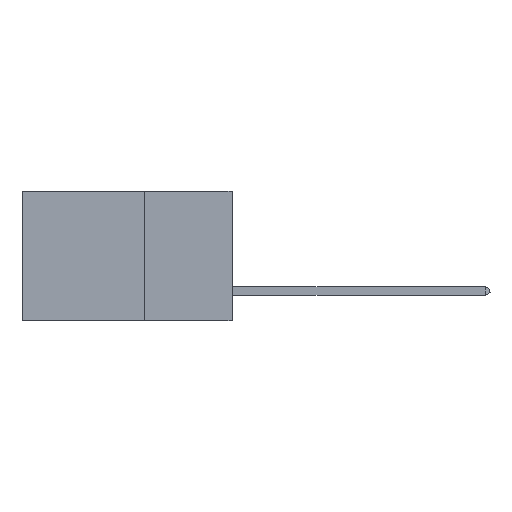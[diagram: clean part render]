
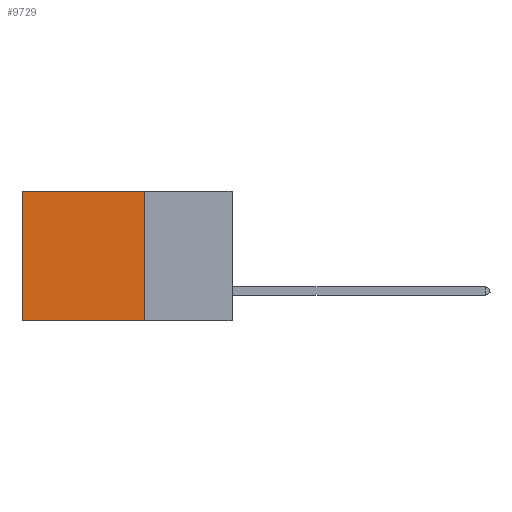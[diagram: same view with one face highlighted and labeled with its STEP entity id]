
A CAD part, left-side view. The second image highlights one B-rep face of the part: STEP entity #9729.
In plain terms, the highlighted planar face has unit normal (-1, 0, 0).
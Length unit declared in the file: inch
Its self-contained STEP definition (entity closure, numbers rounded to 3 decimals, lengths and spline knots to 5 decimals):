
#268 = VERTEX_POINT ( 'NONE', #613 ) ;
#613 = CARTESIAN_POINT ( 'NONE',  ( 0.2875, 0.6, 0. ) ) ;
#1703 = VERTEX_POINT ( 'NONE', #13849 ) ;
#1802 = CARTESIAN_POINT ( 'NONE',  ( 0.2875, 0.6, 0. ) ) ;
#2017 = CARTESIAN_POINT ( 'NONE',  ( 0.2875, 0.25, 0. ) ) ;
#2115 = AXIS2_PLACEMENT_3D ( 'NONE', #5458, #5613, #15082 ) ;
#3708 = VECTOR ( 'NONE', #10103, 39.37008 ) ;
#4011 = ORIENTED_EDGE ( 'NONE', *, *, #12187, .F. ) ;
#4267 = DIRECTION ( 'NONE',  ( 0., 1., 0. ) ) ;
#4859 = VECTOR ( 'NONE', #15124, 39.37008 ) ;
#5458 = CARTESIAN_POINT ( 'NONE',  ( 0.2875, 0.25, 0. ) ) ;
#5613 = DIRECTION ( 'NONE',  ( 1., 0., 0. ) ) ;
#6941 = VERTEX_POINT ( 'NONE', #2017 ) ;
#7247 = LINE ( 'NONE', #11249, #3708 ) ;
#8371 = VECTOR ( 'NONE', #4267, 39.37008 ) ;
#8663 = LINE ( 'NONE', #12694, #11103 ) ;
#8962 = EDGE_CURVE ( 'NONE', #6941, #11988, #8663, .T. ) ;
#9342 = ORIENTED_EDGE ( 'NONE', *, *, #12696, .T. ) ;
#9729 = ADVANCED_FACE ( 'NONE', ( #14822 ), #15032, .F. ) ;
#10103 = DIRECTION ( 'NONE',  ( 0., 1., 0. ) ) ;
#11071 = EDGE_CURVE ( 'NONE', #268, #1703, #13438, .T. ) ;
#11103 = VECTOR ( 'NONE', #15114, 39.37008 ) ;
#11126 = EDGE_LOOP ( 'NONE', ( #14970, #4011, #13406, #9342 ) ) ;
#11249 = CARTESIAN_POINT ( 'NONE',  ( 0.2875, 0.25, 0. ) ) ;
#11988 = VERTEX_POINT ( 'NONE', #14622 ) ;
#12187 = EDGE_CURVE ( 'NONE', #11988, #1703, #14929, .T. ) ;
#12694 = CARTESIAN_POINT ( 'NONE',  ( 0.2875, 0.25, 0. ) ) ;
#12696 = EDGE_CURVE ( 'NONE', #6941, #268, #7247, .T. ) ;
#13406 = ORIENTED_EDGE ( 'NONE', *, *, #8962, .F. ) ;
#13438 = LINE ( 'NONE', #1802, #4859 ) ;
#13849 = CARTESIAN_POINT ( 'NONE',  ( 0.2875, 0.6, -0.37 ) ) ;
#14622 = CARTESIAN_POINT ( 'NONE',  ( 0.2875, 0.25, -0.37 ) ) ;
#14822 = FACE_OUTER_BOUND ( 'NONE', #11126, .T. ) ;
#14929 = LINE ( 'NONE', #15088, #8371 ) ;
#14970 = ORIENTED_EDGE ( 'NONE', *, *, #11071, .T. ) ;
#15032 = PLANE ( 'NONE',  #2115 ) ;
#15082 = DIRECTION ( 'NONE',  ( 0., 0., -1. ) ) ;
#15088 = CARTESIAN_POINT ( 'NONE',  ( 0.2875, 0.25, -0.37 ) ) ;
#15114 = DIRECTION ( 'NONE',  ( 0., 0., -1. ) ) ;
#15124 = DIRECTION ( 'NONE',  ( 0., 0., -1. ) ) ;
